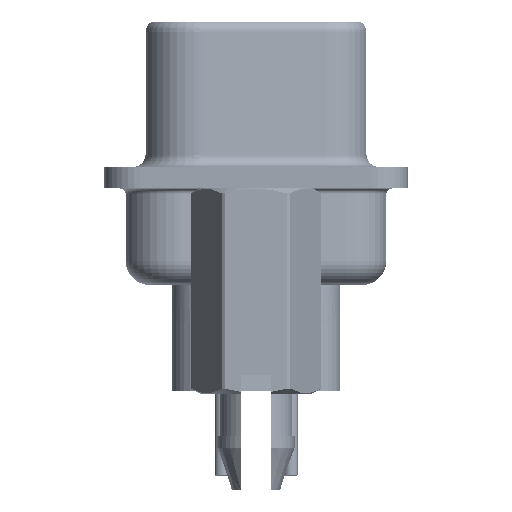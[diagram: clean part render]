
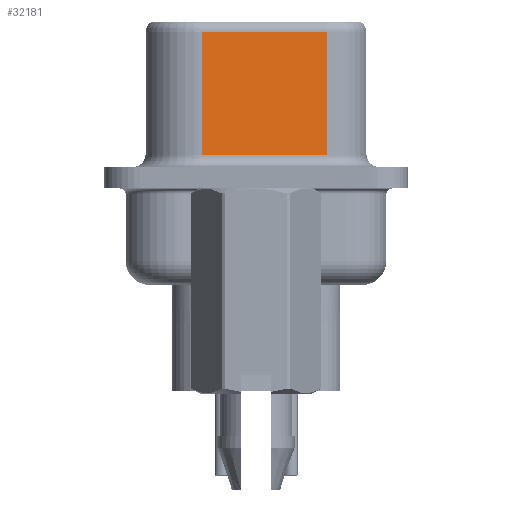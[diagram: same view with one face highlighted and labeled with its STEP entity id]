
A CAD part, left-side view. The second image highlights one B-rep face of the part: STEP entity #32181.
In plain terms, the highlighted planar face has unit normal (-0.985, -0.174, 0).
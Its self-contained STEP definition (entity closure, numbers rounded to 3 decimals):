
#27 = FACE_OUTER_BOUND ( 'NONE', #31379, .T. ) ;
#850 = VERTEX_POINT ( 'NONE', #5006 ) ;
#1359 = EDGE_CURVE ( 'NONE', #49013, #40605, #7942, .T. ) ;
#4448 = DIRECTION ( 'NONE',  ( -0.174, 0.985, 0. ) ) ;
#5006 = CARTESIAN_POINT ( 'NONE',  ( 3.67, 2.233, 0.95 ) ) ;
#5437 = AXIS2_PLACEMENT_3D ( 'NONE', #46340, #12280, #15271 ) ;
#7942 = LINE ( 'NONE', #23157, #31312 ) ;
#8572 = LINE ( 'NONE', #39195, #33300 ) ;
#8913 = CARTESIAN_POINT ( 'NONE',  ( 4.58, -2.927, 6.02 ) ) ;
#11811 = EDGE_CURVE ( 'NONE', #850, #35553, #8572, .T. ) ;
#11913 = LINE ( 'NONE', #46971, #18344 ) ;
#12280 = DIRECTION ( 'NONE',  ( 0.985, 0.174, 0. ) ) ;
#15271 = DIRECTION ( 'NONE',  ( -0.174, 0.985, 0. ) ) ;
#15921 = EDGE_CURVE ( 'NONE', #49013, #35553, #32893, .T. ) ;
#18239 = CARTESIAN_POINT ( 'NONE',  ( 4.58, -2.927, 6.52 ) ) ;
#18344 = VECTOR ( 'NONE', #20608, 1000. ) ;
#20031 = VECTOR ( 'NONE', #33391, 1000. ) ;
#20608 = DIRECTION ( 'NONE',  ( 0., 0., -1. ) ) ;
#22585 = CARTESIAN_POINT ( 'NONE',  ( 3.67, 2.233, 6.02 ) ) ;
#23157 = CARTESIAN_POINT ( 'NONE',  ( 4.58, -2.927, 6.02 ) ) ;
#25747 = ORIENTED_EDGE ( 'NONE', *, *, #1359, .T. ) ;
#31312 = VECTOR ( 'NONE', #4448, 1000. ) ;
#31379 = EDGE_LOOP ( 'NONE', ( #36647, #25747, #37615, #41602 ) ) ;
#32181 = ADVANCED_FACE ( 'NONE', ( #27 ), #37656, .F. ) ;
#32893 = LINE ( 'NONE', #18239, #20031 ) ;
#33300 = VECTOR ( 'NONE', #42680, 1000. ) ;
#33391 = DIRECTION ( 'NONE',  ( 0., 0., -1. ) ) ;
#35553 = VERTEX_POINT ( 'NONE', #46560 ) ;
#36647 = ORIENTED_EDGE ( 'NONE', *, *, #15921, .F. ) ;
#37206 = EDGE_CURVE ( 'NONE', #40605, #850, #11913, .T. ) ;
#37615 = ORIENTED_EDGE ( 'NONE', *, *, #37206, .T. ) ;
#37656 = PLANE ( 'NONE',  #5437 ) ;
#39195 = CARTESIAN_POINT ( 'NONE',  ( 4.58, -2.927, 0.95 ) ) ;
#40605 = VERTEX_POINT ( 'NONE', #22585 ) ;
#41602 = ORIENTED_EDGE ( 'NONE', *, *, #11811, .T. ) ;
#42680 = DIRECTION ( 'NONE',  ( 0.174, -0.985, 0. ) ) ;
#46340 = CARTESIAN_POINT ( 'NONE',  ( 4.58, -2.927, 6.52 ) ) ;
#46560 = CARTESIAN_POINT ( 'NONE',  ( 4.58, -2.927, 0.95 ) ) ;
#46971 = CARTESIAN_POINT ( 'NONE',  ( 3.67, 2.233, 6.52 ) ) ;
#49013 = VERTEX_POINT ( 'NONE', #8913 ) ;
